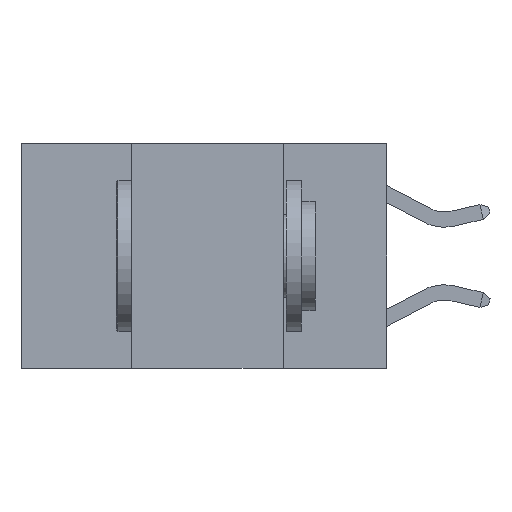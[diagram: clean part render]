
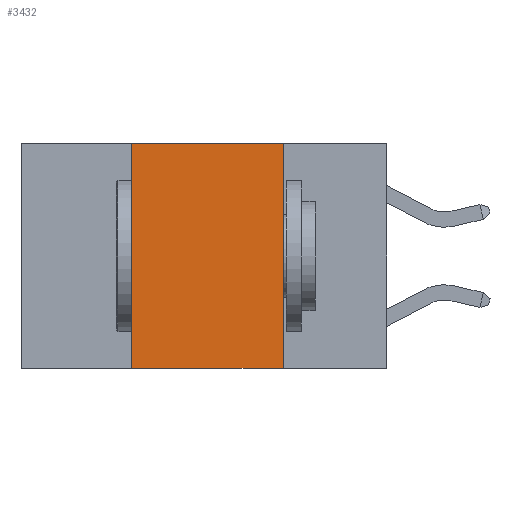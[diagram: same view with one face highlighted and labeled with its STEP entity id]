
A CAD part, left-side view. The second image highlights one B-rep face of the part: STEP entity #3432.
In plain terms, the highlighted planar face has unit normal (-1, 0, 0).
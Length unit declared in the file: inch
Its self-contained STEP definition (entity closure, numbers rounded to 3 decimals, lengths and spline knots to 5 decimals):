
#380 = CARTESIAN_POINT ( 'NONE',  ( 0., 0.42, 0. ) ) ;
#389 = DIRECTION ( 'NONE',  ( 0., 0., -1. ) ) ;
#809 = CARTESIAN_POINT ( 'NONE',  ( 0., 0.42, 0. ) ) ;
#1724 = DIRECTION ( 'NONE',  ( 0., 0., -1. ) ) ;
#1827 = PLANE ( 'NONE',  #4910 ) ;
#2181 = EDGE_CURVE ( 'NONE', #11380, #2351, #14922, .T. ) ;
#2351 = VERTEX_POINT ( 'NONE', #16643 ) ;
#2607 = VECTOR ( 'NONE', #10256, 39.37008 ) ;
#2824 = VECTOR ( 'NONE', #7894, 39.37008 ) ;
#2984 = LINE ( 'NONE', #10130, #9341 ) ;
#3162 = CARTESIAN_POINT ( 'NONE',  ( 0., 0.6, 0. ) ) ;
#3432 = ADVANCED_FACE ( 'NONE', ( #9077 ), #1827, .F. ) ;
#4340 = CARTESIAN_POINT ( 'NONE',  ( 0., 0.17, -0.37 ) ) ;
#4910 = AXIS2_PLACEMENT_3D ( 'NONE', #5010, #13602, #389 ) ;
#5010 = CARTESIAN_POINT ( 'NONE',  ( 0., 0.6, 0. ) ) ;
#5707 = ORIENTED_EDGE ( 'NONE', *, *, #13706, .F. ) ;
#5917 = LINE ( 'NONE', #18549, #2607 ) ;
#6329 = VERTEX_POINT ( 'NONE', #8224 ) ;
#7017 = VECTOR ( 'NONE', #14824, 39.37008 ) ;
#7894 = DIRECTION ( 'NONE',  ( 0., 0., 1. ) ) ;
#8086 = LINE ( 'NONE', #380, #2824 ) ;
#8224 = CARTESIAN_POINT ( 'NONE',  ( 0., 0.42, -0.37 ) ) ;
#9077 = FACE_OUTER_BOUND ( 'NONE', #16245, .T. ) ;
#9341 = VECTOR ( 'NONE', #1724, 39.37008 ) ;
#10130 = CARTESIAN_POINT ( 'NONE',  ( 0., 0.17, 0. ) ) ;
#10256 = DIRECTION ( 'NONE',  ( 0., -1., 0. ) ) ;
#11380 = VERTEX_POINT ( 'NONE', #809 ) ;
#11900 = EDGE_CURVE ( 'NONE', #6329, #11380, #8086, .T. ) ;
#12452 = VERTEX_POINT ( 'NONE', #4340 ) ;
#13018 = ORIENTED_EDGE ( 'NONE', *, *, #17694, .T. ) ;
#13602 = DIRECTION ( 'NONE',  ( 1., 0., 0. ) ) ;
#13706 = EDGE_CURVE ( 'NONE', #2351, #12452, #2984, .T. ) ;
#14345 = ORIENTED_EDGE ( 'NONE', *, *, #11900, .F. ) ;
#14824 = DIRECTION ( 'NONE',  ( 0., -1., 0. ) ) ;
#14922 = LINE ( 'NONE', #3162, #7017 ) ;
#16245 = EDGE_LOOP ( 'NONE', ( #5707, #17340, #14345, #13018 ) ) ;
#16643 = CARTESIAN_POINT ( 'NONE',  ( 0., 0.17, 0. ) ) ;
#17340 = ORIENTED_EDGE ( 'NONE', *, *, #2181, .F. ) ;
#17694 = EDGE_CURVE ( 'NONE', #6329, #12452, #5917, .T. ) ;
#18549 = CARTESIAN_POINT ( 'NONE',  ( 0., 0.6, -0.37 ) ) ;
